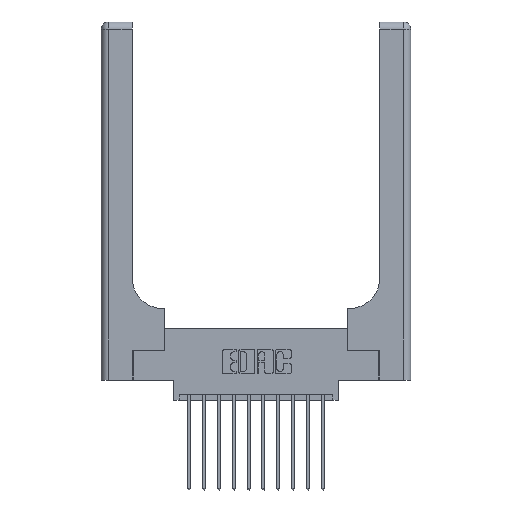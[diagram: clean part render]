
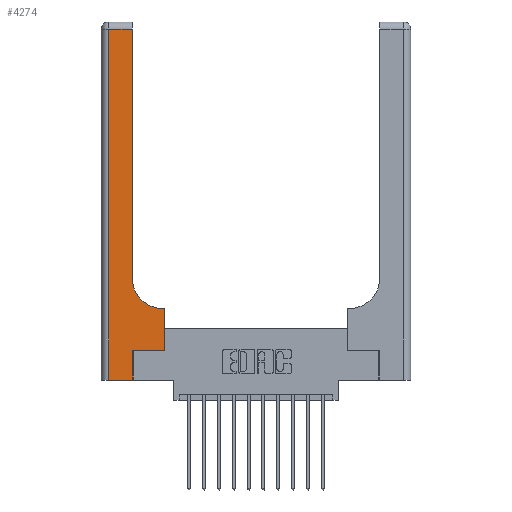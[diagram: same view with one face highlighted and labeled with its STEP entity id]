
A CAD part, top view. The second image highlights one B-rep face of the part: STEP entity #4274.
In plain terms, the highlighted planar face has unit normal (0, 0, 1).
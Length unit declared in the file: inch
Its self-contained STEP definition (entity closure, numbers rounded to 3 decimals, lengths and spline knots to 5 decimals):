
#101 = ORIENTED_EDGE ( 'NONE', *, *, #16049, .T. ) ;
#254 = VERTEX_POINT ( 'NONE', #10563 ) ;
#284 = DIRECTION ( 'NONE',  ( 0., 1., 0. ) ) ;
#291 = VERTEX_POINT ( 'NONE', #314 ) ;
#314 = CARTESIAN_POINT ( 'NONE',  ( 0.51, 0.6, 0.37 ) ) ;
#406 = VECTOR ( 'NONE', #4477, 39.37008 ) ;
#688 = ORIENTED_EDGE ( 'NONE', *, *, #11052, .T. ) ;
#749 = DIRECTION ( 'NONE',  ( -1., 0., 0. ) ) ;
#2017 = CARTESIAN_POINT ( 'NONE',  ( 0., 3., 0.37 ) ) ;
#2025 = VERTEX_POINT ( 'NONE', #3853 ) ;
#2724 = VERTEX_POINT ( 'NONE', #13988 ) ;
#3289 = CARTESIAN_POINT ( 'NONE',  ( 0.265, 0., 0.37 ) ) ;
#3307 = DIRECTION ( 'NONE',  ( 0., 0., -1. ) ) ;
#3448 = LINE ( 'NONE', #9024, #6377 ) ;
#3579 = VERTEX_POINT ( 'NONE', #10303 ) ;
#3853 = CARTESIAN_POINT ( 'NONE',  ( 0.265, 0.25, 0.37 ) ) ;
#4084 = VECTOR ( 'NONE', #6188, 39.37008 ) ;
#4134 = CARTESIAN_POINT ( 'NONE',  ( 0.26, 0.85, 0.37 ) ) ;
#4274 = ADVANCED_FACE ( 'NONE', ( #6592 ), #9519, .F. ) ;
#4477 = DIRECTION ( 'NONE',  ( 0., 1., 0. ) ) ;
#4764 = VERTEX_POINT ( 'NONE', #15565 ) ;
#4876 = DIRECTION ( 'NONE',  ( 0., 1., 0. ) ) ;
#5216 = LINE ( 'NONE', #13651, #14780 ) ;
#5304 = LINE ( 'NONE', #10972, #11555 ) ;
#5715 = LINE ( 'NONE', #9522, #15682 ) ;
#5953 = DIRECTION ( 'NONE',  ( 0., 0., -1. ) ) ;
#6051 = EDGE_CURVE ( 'NONE', #2724, #14582, #8154, .T. ) ;
#6188 = DIRECTION ( 'NONE',  ( 1., 0., 0. ) ) ;
#6377 = VECTOR ( 'NONE', #284, 39.37008 ) ;
#6592 = FACE_OUTER_BOUND ( 'NONE', #10878, .T. ) ;
#6769 = LINE ( 'NONE', #14426, #13052 ) ;
#7154 = AXIS2_PLACEMENT_3D ( 'NONE', #13480, #5953, #14697 ) ;
#7196 = CARTESIAN_POINT ( 'NONE',  ( 0., 2.94, 0.37 ) ) ;
#7200 = ORIENTED_EDGE ( 'NONE', *, *, #6051, .T. ) ;
#7376 = CIRCLE ( 'NONE', #7154, 0.25 ) ;
#8136 = EDGE_CURVE ( 'NONE', #2025, #12297, #6769, .T. ) ;
#8154 = LINE ( 'NONE', #12412, #4084 ) ;
#8228 = ORIENTED_EDGE ( 'NONE', *, *, #11389, .T. ) ;
#8633 = EDGE_CURVE ( 'NONE', #12297, #4764, #3448, .T. ) ;
#8908 = ORIENTED_EDGE ( 'NONE', *, *, #10395, .T. ) ;
#9024 = CARTESIAN_POINT ( 'NONE',  ( 0.528, 0.25, 0.37 ) ) ;
#9374 = EDGE_CURVE ( 'NONE', #3579, #254, #9848, .T. ) ;
#9519 = PLANE ( 'NONE',  #11875 ) ;
#9522 = CARTESIAN_POINT ( 'NONE',  ( 0.26, 0.6, 0.37 ) ) ;
#9848 = LINE ( 'NONE', #7196, #16111 ) ;
#10023 = ORIENTED_EDGE ( 'NONE', *, *, #8136, .T. ) ;
#10303 = CARTESIAN_POINT ( 'NONE',  ( 0.26, 2.94, 0.37 ) ) ;
#10395 = EDGE_CURVE ( 'NONE', #4764, #291, #5715, .T. ) ;
#10454 = CARTESIAN_POINT ( 'NONE',  ( 0.528, 0.25, 0.37 ) ) ;
#10563 = CARTESIAN_POINT ( 'NONE',  ( 0.06, 2.94, 0.37 ) ) ;
#10878 = EDGE_LOOP ( 'NONE', ( #101, #15398, #8228, #7200, #688, #10023, #15661, #8908, #11456 ) ) ;
#10972 = CARTESIAN_POINT ( 'NONE',  ( 0.06, 3., 0.37 ) ) ;
#11052 = EDGE_CURVE ( 'NONE', #14582, #2025, #13752, .T. ) ;
#11389 = EDGE_CURVE ( 'NONE', #254, #2724, #5304, .T. ) ;
#11456 = ORIENTED_EDGE ( 'NONE', *, *, #14600, .T. ) ;
#11555 = VECTOR ( 'NONE', #15133, 39.37008 ) ;
#11875 = AXIS2_PLACEMENT_3D ( 'NONE', #2017, #3307, #12039 ) ;
#12039 = DIRECTION ( 'NONE',  ( -1., 0., 0. ) ) ;
#12265 = VERTEX_POINT ( 'NONE', #4134 ) ;
#12297 = VERTEX_POINT ( 'NONE', #10454 ) ;
#12412 = CARTESIAN_POINT ( 'NONE',  ( 0., 0., 0.37 ) ) ;
#13052 = VECTOR ( 'NONE', #15666, 39.37008 ) ;
#13480 = CARTESIAN_POINT ( 'NONE',  ( 0.51, 0.85, 0.37 ) ) ;
#13651 = CARTESIAN_POINT ( 'NONE',  ( 0.26, 3., 0.37 ) ) ;
#13752 = LINE ( 'NONE', #3289, #406 ) ;
#13988 = CARTESIAN_POINT ( 'NONE',  ( 0.06, 0., 0.37 ) ) ;
#14426 = CARTESIAN_POINT ( 'NONE',  ( 0.265, 0.25, 0.37 ) ) ;
#14582 = VERTEX_POINT ( 'NONE', #15904 ) ;
#14600 = EDGE_CURVE ( 'NONE', #291, #12265, #7376, .T. ) ;
#14697 = DIRECTION ( 'NONE',  ( 1., 0., 0. ) ) ;
#14780 = VECTOR ( 'NONE', #4876, 39.37008 ) ;
#15133 = DIRECTION ( 'NONE',  ( 0., -1., 0. ) ) ;
#15398 = ORIENTED_EDGE ( 'NONE', *, *, #9374, .T. ) ;
#15565 = CARTESIAN_POINT ( 'NONE',  ( 0.528, 0.6, 0.37 ) ) ;
#15661 = ORIENTED_EDGE ( 'NONE', *, *, #8633, .T. ) ;
#15666 = DIRECTION ( 'NONE',  ( 1., 0., 0. ) ) ;
#15682 = VECTOR ( 'NONE', #749, 39.37008 ) ;
#15904 = CARTESIAN_POINT ( 'NONE',  ( 0.265, 0., 0.37 ) ) ;
#15958 = DIRECTION ( 'NONE',  ( -1., 0., 0. ) ) ;
#16049 = EDGE_CURVE ( 'NONE', #12265, #3579, #5216, .T. ) ;
#16111 = VECTOR ( 'NONE', #15958, 39.37008 ) ;
